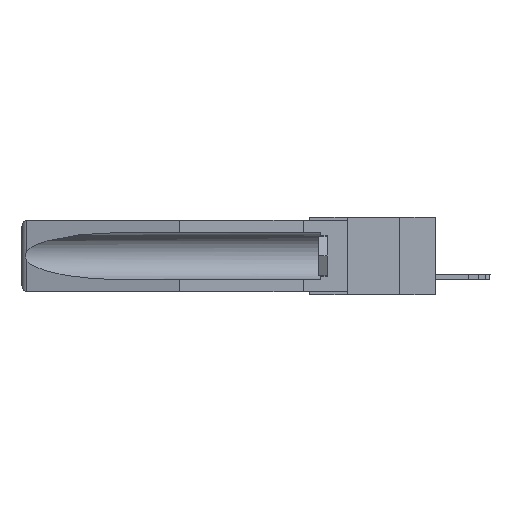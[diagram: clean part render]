
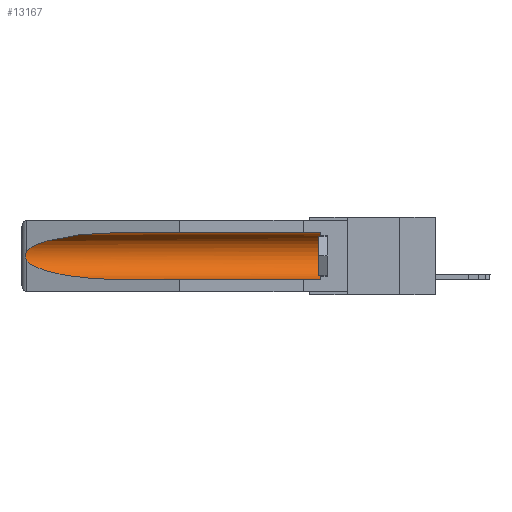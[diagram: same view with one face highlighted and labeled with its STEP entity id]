
A CAD part, left-side view. The second image highlights one B-rep face of the part: STEP entity #13167.
In plain terms, the highlighted cylindrical face has radius 2.857 mm (diameter 5.715 mm), a partial arc.
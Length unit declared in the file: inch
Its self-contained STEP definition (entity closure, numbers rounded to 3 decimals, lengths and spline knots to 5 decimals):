
#1060 = CARTESIAN_POINT ( 'NONE',  ( 0.2675, 1.53308, -0.16763 ) ) ;
#1124 = CARTESIAN_POINT ( 'NONE',  ( 0.26597, 1.52961, -0.15275 ) ) ;
#1624 = VERTEX_POINT ( 'NONE', #13971 ) ;
#1691 = AXIS2_PLACEMENT_3D ( 'NONE', #13564, #13381, #7795 ) ;
#1929 = CARTESIAN_POINT ( 'NONE',  ( 0.26537, 1.52718, -0.14972 ) ) ;
#2299 = EDGE_CURVE ( 'NONE', #7542, #16600, #2705, .T. ) ;
#2609 = CARTESIAN_POINT ( 'NONE',  ( 0.26597, 1.5296, -0.19026 ) ) ;
#2705 = LINE ( 'NONE', #17458, #6203 ) ;
#2916 = VECTOR ( 'NONE', #3333, 39.37008 ) ;
#3091 = VERTEX_POINT ( 'NONE', #15108 ) ;
#3333 = DIRECTION ( 'NONE',  ( 0., 1., 0. ) ) ;
#3586 = DIRECTION ( 'NONE',  ( 0., -1., 0. ) ) ;
#4109 = ORIENTED_EDGE ( 'NONE', *, *, #10344, .T. ) ;
#4329 = CARTESIAN_POINT ( 'NONE',  ( 0.25451, 1.48313, -0.09465 ) ) ;
#4612 = CARTESIAN_POINT ( 'NONE',  ( 0.21114, 1.30732, -0.284 ) ) ;
#4745 = CARTESIAN_POINT ( 'NONE',  ( 0.26537, 1.52718, -0.19328 ) ) ;
#5188 =( BOUNDED_CURVE ( )  B_SPLINE_CURVE ( 3, ( #4745, #6050, #4612, #9214 ),
 .UNSPECIFIED., .F., .F. ) 
 B_SPLINE_CURVE_WITH_KNOTS ( ( 4, 4 ),
 ( 0.1948, 1.5708 ),
 .UNSPECIFIED. ) 
 CURVE ( )  GEOMETRIC_REPRESENTATION_ITEM ( )  RATIONAL_B_SPLINE_CURVE ( ( 1., 0.848, 0.848, 1. ) ) 
 REPRESENTATION_ITEM ( '' )  );
#5265 = CARTESIAN_POINT ( 'NONE',  ( 0.26537, 1.52718, -0.19328 ) ) ;
#5339 = ORIENTED_EDGE ( 'NONE', *, *, #13634, .T. ) ;
#5464 = ORIENTED_EDGE ( 'NONE', *, *, #15035, .T. ) ;
#5538 = CARTESIAN_POINT ( 'NONE',  ( 0.2673, 1.5327, -0.16383 ) ) ;
#5624 = CARTESIAN_POINT ( 'NONE',  ( 0.155, 1.07973, -0.284 ) ) ;
#5645 = CARTESIAN_POINT ( 'NONE',  ( 0.155, 1.07973, -0.059 ) ) ;
#5716 = LINE ( 'NONE', #13482, #2916 ) ;
#6050 = CARTESIAN_POINT ( 'NONE',  ( 0.25451, 1.48313, -0.24835 ) ) ;
#6203 = VECTOR ( 'NONE', #14577, 39.37008 ) ;
#7172 = CARTESIAN_POINT ( 'NONE',  ( 0.2673, 1.53269, -0.17917 ) ) ;
#7216 = CARTESIAN_POINT ( 'NONE',  ( 0.21114, 1.30732, -0.059 ) ) ;
#7542 = VERTEX_POINT ( 'NONE', #19007 ) ;
#7795 = DIRECTION ( 'NONE',  ( 0., 0., 1. ) ) ;
#8649 = CARTESIAN_POINT ( 'NONE',  ( 0.26537, 1.52718, -0.19328 ) ) ;
#9214 = CARTESIAN_POINT ( 'NONE',  ( 0.155, 1.07973, -0.284 ) ) ;
#10066 = VERTEX_POINT ( 'NONE', #1929 ) ;
#10271 = VERTEX_POINT ( 'NONE', #5265 ) ;
#10344 = EDGE_CURVE ( 'NONE', #10066, #10271, #11668, .T. ) ;
#11198 = EDGE_CURVE ( 'NONE', #7542, #1624, #16087, .T. ) ;
#11573 = ORIENTED_EDGE ( 'NONE', *, *, #11198, .T. ) ;
#11668 = B_SPLINE_CURVE_WITH_KNOTS ( 'NONE', 3,
 ( #14355, #1124, #14227, #5538, #1060, #15875, #7172, #15731, #2609, #8649 ),
 .UNSPECIFIED., .F., .F.,
 ( 4, 2, 2, 2, 4 ),
 ( 0., 0.00029, 0.00058, 0.00087, 0.00117 ),
 .UNSPECIFIED. ) ;
#11819 = FACE_OUTER_BOUND ( 'NONE', #16320, .T. ) ;
#12008 =( BOUNDED_CURVE ( )  B_SPLINE_CURVE ( 3, ( #5645, #7216, #4329, #18798 ),
 .UNSPECIFIED., .F., .F. ) 
 B_SPLINE_CURVE_WITH_KNOTS ( ( 4, 4 ),
 ( 4.71239, 6.08839 ),
 .UNSPECIFIED. ) 
 CURVE ( )  GEOMETRIC_REPRESENTATION_ITEM ( )  RATIONAL_B_SPLINE_CURVE ( ( 1., 0.848, 0.848, 1. ) ) 
 REPRESENTATION_ITEM ( '' )  );
#12157 = ORIENTED_EDGE ( 'NONE', *, *, #17438, .T. ) ;
#12478 = CYLINDRICAL_SURFACE ( 'NONE', #1691, 0.1125 ) ;
#13167 = ADVANCED_FACE ( 'NONE', ( #11819 ), #12478, .F. ) ;
#13381 = DIRECTION ( 'NONE',  ( 0., 1., 0. ) ) ;
#13482 = CARTESIAN_POINT ( 'NONE',  ( 0.155, -0.30754, -0.059 ) ) ;
#13564 = CARTESIAN_POINT ( 'NONE',  ( 0.155, -0.30754, -0.1715 ) ) ;
#13634 = EDGE_CURVE ( 'NONE', #3091, #10066, #12008, .T. ) ;
#13971 = CARTESIAN_POINT ( 'NONE',  ( 0.155, 0.126, -0.059 ) ) ;
#14227 = CARTESIAN_POINT ( 'NONE',  ( 0.26654, 1.53092, -0.15636 ) ) ;
#14355 = CARTESIAN_POINT ( 'NONE',  ( 0.26537, 1.52718, -0.14972 ) ) ;
#14577 = DIRECTION ( 'NONE',  ( 0., 1., 0. ) ) ;
#14695 = ORIENTED_EDGE ( 'NONE', *, *, #2299, .F. ) ;
#15035 = EDGE_CURVE ( 'NONE', #10271, #16600, #5188, .T. ) ;
#15108 = CARTESIAN_POINT ( 'NONE',  ( 0.155, 1.07973, -0.059 ) ) ;
#15731 = CARTESIAN_POINT ( 'NONE',  ( 0.26655, 1.53094, -0.18657 ) ) ;
#15875 = CARTESIAN_POINT ( 'NONE',  ( 0.2675, 1.53308, -0.17534 ) ) ;
#16087 = CIRCLE ( 'NONE', #18992, 0.1125 ) ;
#16320 = EDGE_LOOP ( 'NONE', ( #5339, #4109, #5464, #14695, #11573, #12157 ) ) ;
#16600 = VERTEX_POINT ( 'NONE', #5624 ) ;
#17438 = EDGE_CURVE ( 'NONE', #1624, #3091, #5716, .T. ) ;
#17458 = CARTESIAN_POINT ( 'NONE',  ( 0.155, -0.30754, -0.284 ) ) ;
#18083 = DIRECTION ( 'NONE',  ( 0., 0., 1. ) ) ;
#18146 = CARTESIAN_POINT ( 'NONE',  ( 0.155, 0.126, -0.1715 ) ) ;
#18798 = CARTESIAN_POINT ( 'NONE',  ( 0.26537, 1.52718, -0.14972 ) ) ;
#18992 = AXIS2_PLACEMENT_3D ( 'NONE', #18146, #3586, #18083 ) ;
#19007 = CARTESIAN_POINT ( 'NONE',  ( 0.155, 0.126, -0.284 ) ) ;
